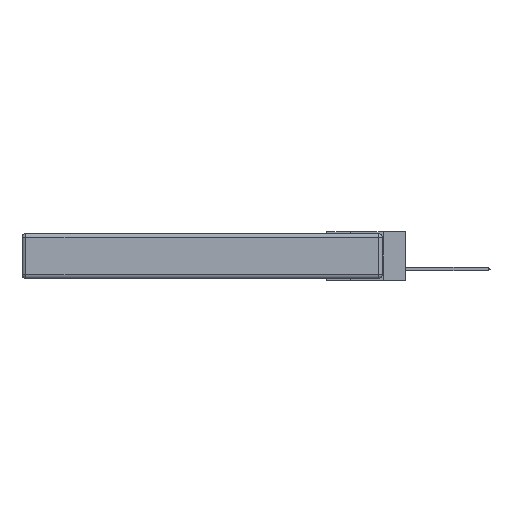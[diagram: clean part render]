
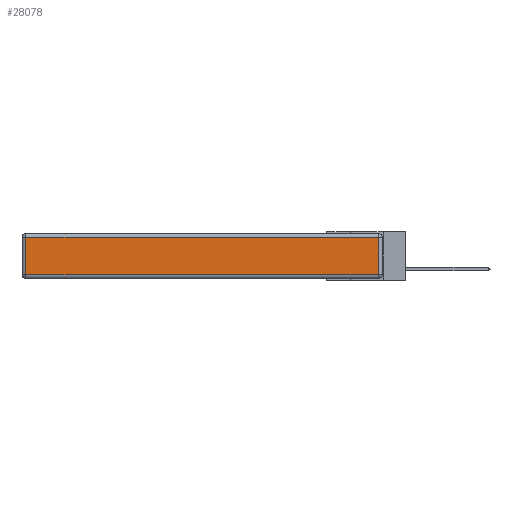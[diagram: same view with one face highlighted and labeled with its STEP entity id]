
A CAD part, left-side view. The second image highlights one B-rep face of the part: STEP entity #28078.
In plain terms, the highlighted planar face has unit normal (-1, 0, 0).
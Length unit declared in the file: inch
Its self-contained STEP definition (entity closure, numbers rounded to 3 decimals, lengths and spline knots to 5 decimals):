
#1148 = LINE ( 'NONE', #6281, #17739 ) ;
#2957 = EDGE_CURVE ( 'NONE', #27534, #10350, #5762, .T. ) ;
#3684 = EDGE_CURVE ( 'NONE', #27855, #6403, #23024, .T. ) ;
#3794 = CARTESIAN_POINT ( 'NONE',  ( 0., 2.72, -0.343 ) ) ;
#4159 = DIRECTION ( 'NONE',  ( 0., 0., 1. ) ) ;
#4326 = DIRECTION ( 'NONE',  ( -1., 0., 0. ) ) ;
#5441 = LINE ( 'NONE', #3794, #12728 ) ;
#5762 = LINE ( 'NONE', #24478, #28581 ) ;
#6281 = CARTESIAN_POINT ( 'NONE',  ( 0., 0.03, -0.343 ) ) ;
#6403 = VERTEX_POINT ( 'NONE', #15484 ) ;
#8181 = DIRECTION ( 'NONE',  ( 0., -1., 0. ) ) ;
#8515 = FACE_OUTER_BOUND ( 'NONE', #28216, .T. ) ;
#8734 = DIRECTION ( 'NONE',  ( 0., 1., 0. ) ) ;
#8762 = DIRECTION ( 'NONE',  ( 0., 0., 1. ) ) ;
#9644 = AXIS2_PLACEMENT_3D ( 'NONE', #10815, #4326, #8762 ) ;
#10350 = VERTEX_POINT ( 'NONE', #11848 ) ;
#10815 = CARTESIAN_POINT ( 'NONE',  ( 0., 0., -0.343 ) ) ;
#11848 = CARTESIAN_POINT ( 'NONE',  ( 0., 2.72, -0.03 ) ) ;
#12728 = VECTOR ( 'NONE', #19214, 39.37008 ) ;
#13685 = VECTOR ( 'NONE', #8181, 39.37008 ) ;
#15437 = PLANE ( 'NONE',  #9644 ) ;
#15484 = CARTESIAN_POINT ( 'NONE',  ( 0., 0.03, -0.313 ) ) ;
#16509 = CARTESIAN_POINT ( 'NONE',  ( 0., 0.03, -0.03 ) ) ;
#17739 = VECTOR ( 'NONE', #4159, 39.37008 ) ;
#18696 = CARTESIAN_POINT ( 'NONE',  ( 0., 2.72, -0.313 ) ) ;
#19214 = DIRECTION ( 'NONE',  ( 0., 0., -1. ) ) ;
#21243 = ORIENTED_EDGE ( 'NONE', *, *, #24838, .T. ) ;
#21729 = CARTESIAN_POINT ( 'NONE',  ( 0., 0., -0.313 ) ) ;
#22017 = EDGE_CURVE ( 'NONE', #10350, #27855, #5441, .T. ) ;
#23024 = LINE ( 'NONE', #21729, #13685 ) ;
#24478 = CARTESIAN_POINT ( 'NONE',  ( 0., 2.75, -0.03 ) ) ;
#24838 = EDGE_CURVE ( 'NONE', #6403, #27534, #1148, .T. ) ;
#25846 = ORIENTED_EDGE ( 'NONE', *, *, #2957, .T. ) ;
#27534 = VERTEX_POINT ( 'NONE', #16509 ) ;
#27599 = ORIENTED_EDGE ( 'NONE', *, *, #3684, .T. ) ;
#27716 = ORIENTED_EDGE ( 'NONE', *, *, #22017, .T. ) ;
#27855 = VERTEX_POINT ( 'NONE', #18696 ) ;
#28078 = ADVANCED_FACE ( 'NONE', ( #8515 ), #15437, .T. ) ;
#28216 = EDGE_LOOP ( 'NONE', ( #27599, #21243, #25846, #27716 ) ) ;
#28581 = VECTOR ( 'NONE', #8734, 39.37008 ) ;
